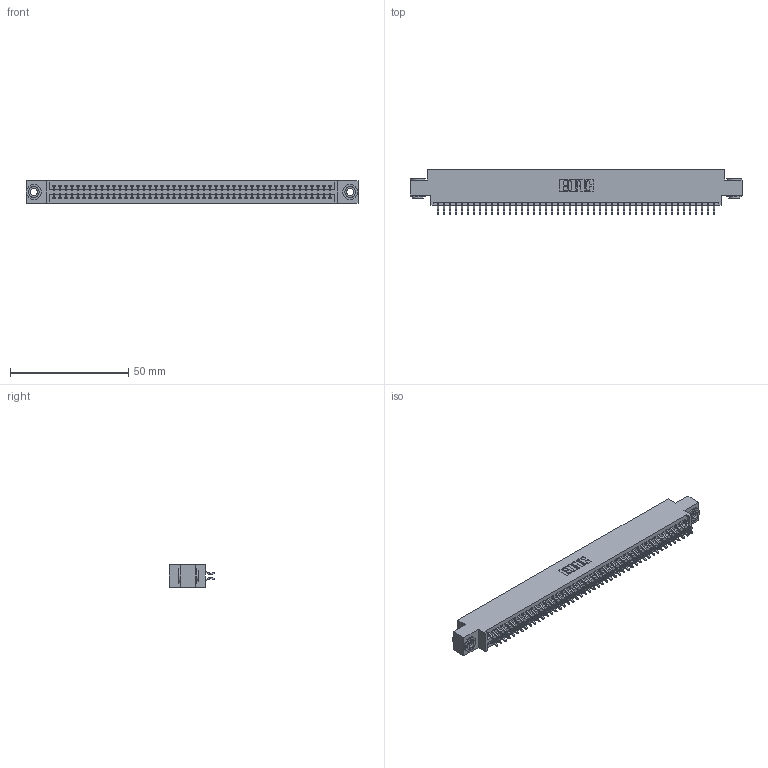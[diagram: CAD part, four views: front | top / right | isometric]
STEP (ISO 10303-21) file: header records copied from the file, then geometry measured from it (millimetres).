
FILE_DESCRIPTION (( 'STEP AP203' ), '1' );
FILE_NAME ('395-094-556-803.STEP', '2019-10-25T22:57:52', ( '' ), ( '' ), 'SwSTEP 2.0', 'SolidWorks 2016', '' );
FILE_SCHEMA (( 'CONFIG_CONTROL_DESIGN' ));
Length unit declared in the file: inch
Products named in the file (4): 345-250-002_345-250-002-102; 395-094-556-803; 345 Part_0.170 Offset - 0.156 Dia-TH; 345-292-001_556 Tail
Assembly tree (97 placements, depth 2):
  395-094-556-803
    345 Part_0.170 Offset - 0.156 Dia-TH
    345-292-001_556 Tail  x94
    345-250-002_345-250-002-102  x2
Bounding box: 140.59 x 19.24 x 9.4 mm (x, y, z)
Volume: 13605.7 mm3; surface area: 20474.4 mm2
Topology: 97 solids, 97 shells, 5432 faces, 16127 edges, 10622 vertices
Faces by surface type: plane 3572, cylinder 1852, cone 8
Entity records: 37206 total; most frequent: CARTESIAN_POINT 6223, ORIENTED_EDGE 6138, DIRECTION 5499, EDGE_CURVE 3069, LINE 2717, VECTOR 2717, VERTEX_POINT 2042, AXIS2_PLACEMENT_3D 1391
